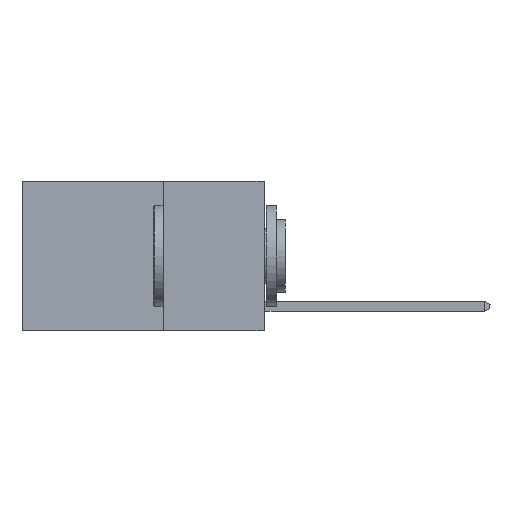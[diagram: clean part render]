
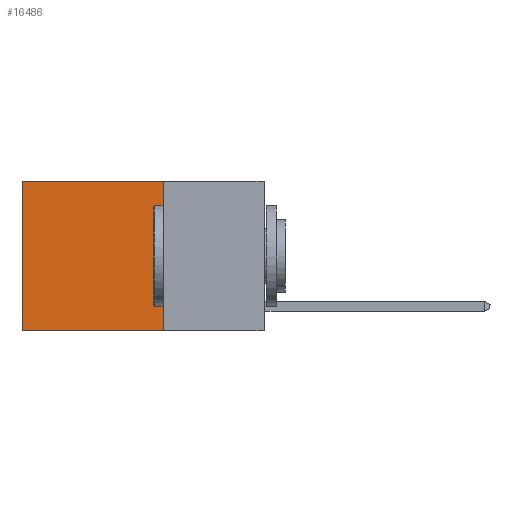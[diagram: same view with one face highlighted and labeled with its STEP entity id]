
A CAD part, left-side view. The second image highlights one B-rep face of the part: STEP entity #16486.
In plain terms, the highlighted planar face has unit normal (-1, 0, 0).
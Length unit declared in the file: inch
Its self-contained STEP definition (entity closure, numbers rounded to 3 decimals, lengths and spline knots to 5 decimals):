
#727 = ORIENTED_EDGE ( 'NONE', *, *, #13854, .T. ) ;
#913 = VERTEX_POINT ( 'NONE', #3084 ) ;
#2474 = DIRECTION ( 'NONE',  ( 0., 1., 0. ) ) ;
#2592 = VERTEX_POINT ( 'NONE', #24742 ) ;
#2649 = EDGE_CURVE ( 'NONE', #12480, #913, #24420, .T. ) ;
#2898 = VECTOR ( 'NONE', #18903, 39.37008 ) ;
#3084 = CARTESIAN_POINT ( 'NONE',  ( 0.2625, 0.6, -0.37 ) ) ;
#3141 = EDGE_LOOP ( 'NONE', ( #16206, #16855, #13050, #727 ) ) ;
#6072 = FACE_OUTER_BOUND ( 'NONE', #3141, .T. ) ;
#6592 = AXIS2_PLACEMENT_3D ( 'NONE', #20514, #10462, #24500 ) ;
#6788 = VECTOR ( 'NONE', #10698, 39.37008 ) ;
#7160 = CARTESIAN_POINT ( 'NONE',  ( 0.2625, 0.25, -0.37 ) ) ;
#8422 = PLANE ( 'NONE',  #6592 ) ;
#8614 = VECTOR ( 'NONE', #24380, 39.37008 ) ;
#8833 = CARTESIAN_POINT ( 'NONE',  ( 0.2625, 0.25, -0.37 ) ) ;
#10462 = DIRECTION ( 'NONE',  ( 1., 0., 0. ) ) ;
#10698 = DIRECTION ( 'NONE',  ( 0., 0., -1. ) ) ;
#12480 = VERTEX_POINT ( 'NONE', #7160 ) ;
#13050 = ORIENTED_EDGE ( 'NONE', *, *, #21530, .F. ) ;
#13854 = EDGE_CURVE ( 'NONE', #2592, #21009, #17322, .T. ) ;
#14623 = LINE ( 'NONE', #20484, #8614 ) ;
#16206 = ORIENTED_EDGE ( 'NONE', *, *, #26029, .T. ) ;
#16486 = ADVANCED_FACE ( 'NONE', ( #6072 ), #8422, .F. ) ;
#16855 = ORIENTED_EDGE ( 'NONE', *, *, #2649, .F. ) ;
#17322 = LINE ( 'NONE', #20775, #17961 ) ;
#17961 = VECTOR ( 'NONE', #2474, 39.37008 ) ;
#18903 = DIRECTION ( 'NONE',  ( 0., 1., 0. ) ) ;
#19229 = CARTESIAN_POINT ( 'NONE',  ( 0.2625, 0.6, 0. ) ) ;
#20484 = CARTESIAN_POINT ( 'NONE',  ( 0.2625, 0.6, 0. ) ) ;
#20514 = CARTESIAN_POINT ( 'NONE',  ( 0.2625, 0.25, 0. ) ) ;
#20741 = CARTESIAN_POINT ( 'NONE',  ( 0.2625, 0.25, 0. ) ) ;
#20775 = CARTESIAN_POINT ( 'NONE',  ( 0.2625, 0.25, 0. ) ) ;
#21009 = VERTEX_POINT ( 'NONE', #19229 ) ;
#21530 = EDGE_CURVE ( 'NONE', #2592, #12480, #22860, .T. ) ;
#22860 = LINE ( 'NONE', #20741, #6788 ) ;
#24380 = DIRECTION ( 'NONE',  ( 0., 0., -1. ) ) ;
#24420 = LINE ( 'NONE', #8833, #2898 ) ;
#24500 = DIRECTION ( 'NONE',  ( 0., 0., -1. ) ) ;
#24742 = CARTESIAN_POINT ( 'NONE',  ( 0.2625, 0.25, 0. ) ) ;
#26029 = EDGE_CURVE ( 'NONE', #21009, #913, #14623, .T. ) ;
